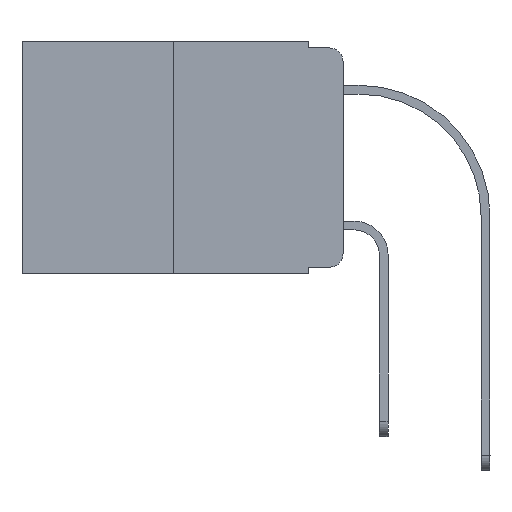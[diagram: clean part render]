
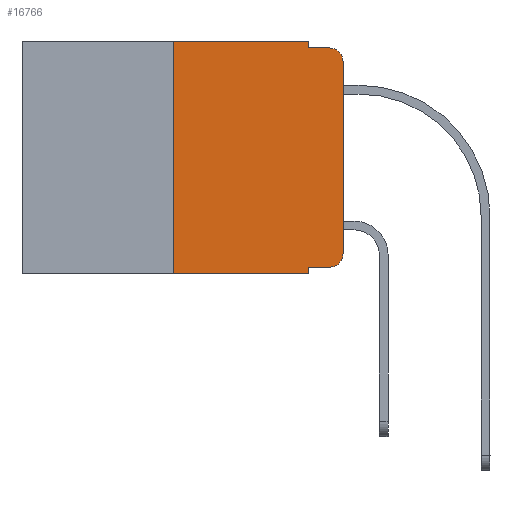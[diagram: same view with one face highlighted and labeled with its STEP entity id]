
A CAD part, left-side view. The second image highlights one B-rep face of the part: STEP entity #16766.
In plain terms, the highlighted planar face has unit normal (-1, 0, 0).
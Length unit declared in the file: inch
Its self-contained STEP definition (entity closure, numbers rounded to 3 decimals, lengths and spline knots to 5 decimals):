
#61 = VERTEX_POINT ( 'NONE', #8952 ) ;
#240 = VECTOR ( 'NONE', #9541, 39.37008 ) ;
#332 = EDGE_CURVE ( 'NONE', #6581, #1274, #6316, .T. ) ;
#506 = VERTEX_POINT ( 'NONE', #10305 ) ;
#933 = ORIENTED_EDGE ( 'NONE', *, *, #2585, .T. ) ;
#1274 = VERTEX_POINT ( 'NONE', #10042 ) ;
#1310 = DIRECTION ( 'NONE',  ( 0., -1., 0. ) ) ;
#1661 = VERTEX_POINT ( 'NONE', #9253 ) ;
#1729 = LINE ( 'NONE', #7706, #9003 ) ;
#1823 = ORIENTED_EDGE ( 'NONE', *, *, #7255, .F. ) ;
#1886 = ORIENTED_EDGE ( 'NONE', *, *, #12633, .F. ) ;
#2003 = CARTESIAN_POINT ( 'NONE',  ( 0., 0.25, 0. ) ) ;
#2200 = VECTOR ( 'NONE', #18658, 39.37008 ) ;
#2483 = DIRECTION ( 'NONE',  ( 0., 0., 1. ) ) ;
#2585 = EDGE_CURVE ( 'NONE', #13281, #61, #16927, .T. ) ;
#2885 = CARTESIAN_POINT ( 'NONE',  ( 0., 0.02, -0.313 ) ) ;
#3047 = CIRCLE ( 'NONE', #10850, 0.02 ) ;
#3051 = EDGE_CURVE ( 'NONE', #506, #1661, #3584, .T. ) ;
#3584 = LINE ( 'NONE', #16904, #240 ) ;
#3975 = VECTOR ( 'NONE', #12702, 39.37008 ) ;
#4473 = CARTESIAN_POINT ( 'NONE',  ( 0., 0.02, -0.03 ) ) ;
#4701 = VECTOR ( 'NONE', #8584, 39.37008 ) ;
#5419 = LINE ( 'NONE', #14500, #12086 ) ;
#5577 = AXIS2_PLACEMENT_3D ( 'NONE', #17593, #11422, #17400 ) ;
#5899 = EDGE_CURVE ( 'NONE', #13633, #6983, #15532, .T. ) ;
#6316 = LINE ( 'NONE', #9345, #8773 ) ;
#6581 = VERTEX_POINT ( 'NONE', #10398 ) ;
#6983 = VERTEX_POINT ( 'NONE', #7432 ) ;
#7255 = EDGE_CURVE ( 'NONE', #506, #1274, #11623, .T. ) ;
#7432 = CARTESIAN_POINT ( 'NONE',  ( 0., 0.02, -0.01 ) ) ;
#7569 = ORIENTED_EDGE ( 'NONE', *, *, #5899, .F. ) ;
#7706 = CARTESIAN_POINT ( 'NONE',  ( 0., 0.051, 0. ) ) ;
#8584 = DIRECTION ( 'NONE',  ( 0., 0., -1. ) ) ;
#8605 = ORIENTED_EDGE ( 'NONE', *, *, #13210, .T. ) ;
#8773 = VECTOR ( 'NONE', #13934, 39.37008 ) ;
#8850 = DIRECTION ( 'NONE',  ( 0., 0., -1. ) ) ;
#8952 = CARTESIAN_POINT ( 'NONE',  ( 0., 0., -0.03 ) ) ;
#9003 = VECTOR ( 'NONE', #16702, 39.37008 ) ;
#9253 = CARTESIAN_POINT ( 'NONE',  ( 0., 0.02, -0.333 ) ) ;
#9345 = CARTESIAN_POINT ( 'NONE',  ( 0., 0.473, -0.343 ) ) ;
#9541 = DIRECTION ( 'NONE',  ( 0., -1., 0. ) ) ;
#9989 = DIRECTION ( 'NONE',  ( -1., 0., 0. ) ) ;
#10042 = CARTESIAN_POINT ( 'NONE',  ( 0., 0.051, -0.343 ) ) ;
#10305 = CARTESIAN_POINT ( 'NONE',  ( 0., 0.051, -0.333 ) ) ;
#10398 = CARTESIAN_POINT ( 'NONE',  ( 0., 0.25, -0.343 ) ) ;
#10559 = EDGE_LOOP ( 'NONE', ( #933, #8605, #7569, #16918, #1886, #12831, #12540, #1823, #14095, #12457 ) ) ;
#10850 = AXIS2_PLACEMENT_3D ( 'NONE', #4473, #9989, #12923 ) ;
#10944 = CARTESIAN_POINT ( 'NONE',  ( 0., 0., 0. ) ) ;
#11050 = EDGE_CURVE ( 'NONE', #1661, #13281, #12348, .T. ) ;
#11422 = DIRECTION ( 'NONE',  ( 1., 0., 0. ) ) ;
#11623 = LINE ( 'NONE', #13183, #4701 ) ;
#12086 = VECTOR ( 'NONE', #2483, 39.37008 ) ;
#12348 = CIRCLE ( 'NONE', #13276, 0.02 ) ;
#12457 = ORIENTED_EDGE ( 'NONE', *, *, #11050, .T. ) ;
#12540 = ORIENTED_EDGE ( 'NONE', *, *, #332, .T. ) ;
#12633 = EDGE_CURVE ( 'NONE', #13858, #14264, #18906, .T. ) ;
#12693 = EDGE_CURVE ( 'NONE', #6581, #13858, #5419, .T. ) ;
#12695 = CARTESIAN_POINT ( 'NONE',  ( 0., 0.051, -0.01 ) ) ;
#12702 = DIRECTION ( 'NONE',  ( 0., 0., 1. ) ) ;
#12831 = ORIENTED_EDGE ( 'NONE', *, *, #12693, .F. ) ;
#12923 = DIRECTION ( 'NONE',  ( 0., 0., -1. ) ) ;
#13093 = FACE_OUTER_BOUND ( 'NONE', #10559, .T. ) ;
#13183 = CARTESIAN_POINT ( 'NONE',  ( 0., 0.051, 0. ) ) ;
#13210 = EDGE_CURVE ( 'NONE', #61, #6983, #3047, .T. ) ;
#13234 = CARTESIAN_POINT ( 'NONE',  ( 0., 0.473, 0. ) ) ;
#13276 = AXIS2_PLACEMENT_3D ( 'NONE', #2885, #15100, #8850 ) ;
#13281 = VERTEX_POINT ( 'NONE', #16617 ) ;
#13633 = VERTEX_POINT ( 'NONE', #17576 ) ;
#13858 = VERTEX_POINT ( 'NONE', #2003 ) ;
#13934 = DIRECTION ( 'NONE',  ( 0., -1., 0. ) ) ;
#14095 = ORIENTED_EDGE ( 'NONE', *, *, #3051, .T. ) ;
#14264 = VERTEX_POINT ( 'NONE', #16576 ) ;
#14500 = CARTESIAN_POINT ( 'NONE',  ( 0., 0.25, 0. ) ) ;
#14551 = PLANE ( 'NONE',  #5577 ) ;
#15100 = DIRECTION ( 'NONE',  ( -1., 0., 0. ) ) ;
#15532 = LINE ( 'NONE', #12695, #2200 ) ;
#16463 = VECTOR ( 'NONE', #1310, 39.37008 ) ;
#16576 = CARTESIAN_POINT ( 'NONE',  ( 0., 0.051, 0. ) ) ;
#16617 = CARTESIAN_POINT ( 'NONE',  ( 0., 0., -0.313 ) ) ;
#16702 = DIRECTION ( 'NONE',  ( 0., 0., -1. ) ) ;
#16766 = ADVANCED_FACE ( 'NONE', ( #13093 ), #14551, .F. ) ;
#16889 = EDGE_CURVE ( 'NONE', #14264, #13633, #1729, .T. ) ;
#16904 = CARTESIAN_POINT ( 'NONE',  ( 0., 0.051, -0.333 ) ) ;
#16918 = ORIENTED_EDGE ( 'NONE', *, *, #16889, .F. ) ;
#16927 = LINE ( 'NONE', #10944, #3975 ) ;
#17400 = DIRECTION ( 'NONE',  ( 0., 0., -1. ) ) ;
#17576 = CARTESIAN_POINT ( 'NONE',  ( 0., 0.051, -0.01 ) ) ;
#17593 = CARTESIAN_POINT ( 'NONE',  ( 0., 0.473, 0. ) ) ;
#18658 = DIRECTION ( 'NONE',  ( 0., -1., 0. ) ) ;
#18906 = LINE ( 'NONE', #13234, #16463 ) ;
